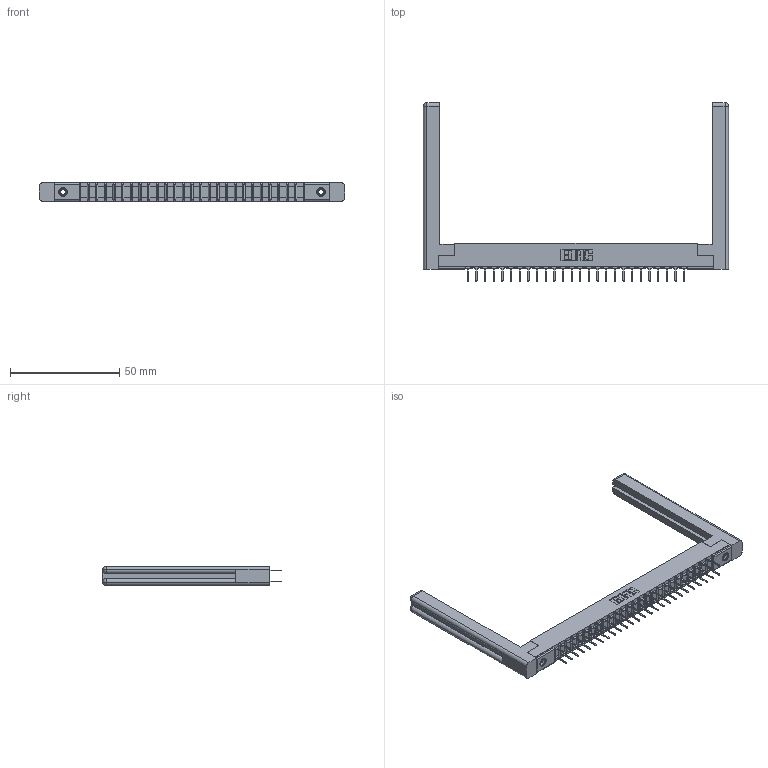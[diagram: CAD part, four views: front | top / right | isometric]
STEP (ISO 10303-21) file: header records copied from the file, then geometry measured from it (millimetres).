
FILE_DESCRIPTION (( 'STEP AP203' ), '1' );
FILE_NAME ('307-052-524-258.STEP', '2019-09-06T12:10:10', ( '' ), ( '' ), 'SwSTEP 2.0', 'SolidWorks 2016', '' );
FILE_SCHEMA (( 'CONFIG_CONTROL_DESIGN' ));
Length unit declared in the file: inch
Products named in the file (5): 345-250-001_345-250-001-102; 307 Part_.156 Dia Mounting Holes; 307-052-524-258; 307-220-058; 307-290-001_524
Assembly tree (57 placements, depth 2):
  307-052-524-258
    307 Part_.156 Dia Mounting Holes
    307-290-001_524  x52
    307-220-058  x2
    345-250-001_345-250-001-102  x2
Bounding box: 139.65 x 81.74 x 8.71 mm (x, y, z)
Volume: 16803.9 mm3; surface area: 21312.8 mm2
Topology: 57 solids, 57 shells, 2679 faces, 7437 edges, 4802 vertices
Faces by surface type: plane 1766, cylinder 835, sphere 54, torus 12, cone 12
Entity records: 27695 total; most frequent: CARTESIAN_POINT 4553, ORIENTED_EDGE 4452, DIRECTION 4424, EDGE_CURVE 2226, LINE 1698, VECTOR 1698, VERTEX_POINT 1438, AXIS2_PLACEMENT_3D 1363
